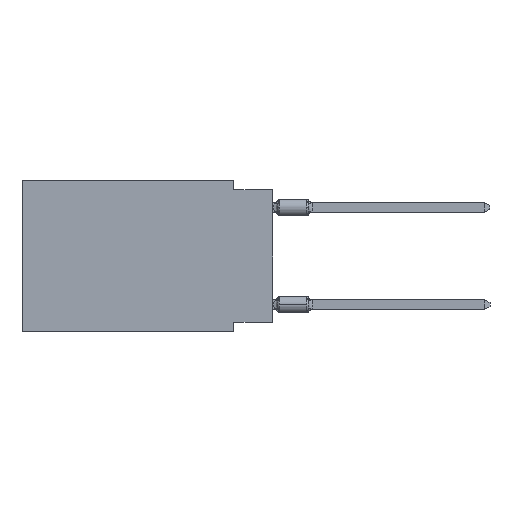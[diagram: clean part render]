
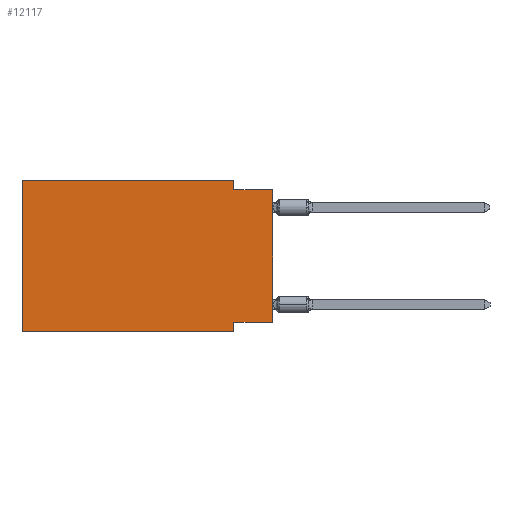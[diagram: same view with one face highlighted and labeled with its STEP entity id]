
A CAD part, left-side view. The second image highlights one B-rep face of the part: STEP entity #12117.
In plain terms, the highlighted planar face has unit normal (-1, 0, 0).
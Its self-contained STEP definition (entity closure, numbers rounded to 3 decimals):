
#54 = VERTEX_POINT ( 'NONE', #26732 ) ;
#307 = VECTOR ( 'NONE', #13949, 1000. ) ;
#312 = CARTESIAN_POINT ( 'NONE',  ( 0., 0., -0.635 ) ) ;
#719 = VERTEX_POINT ( 'NONE', #14793 ) ;
#890 = LINE ( 'NONE', #18001, #26978 ) ;
#1674 = ORIENTED_EDGE ( 'NONE', *, *, #17849, .F. ) ;
#1711 = CARTESIAN_POINT ( 'NONE',  ( 0., 16.383, 0. ) ) ;
#2446 = LINE ( 'NONE', #312, #4805 ) ;
#3516 = DIRECTION ( 'NONE',  ( 0., -1., 0. ) ) ;
#4029 = DIRECTION ( 'NONE',  ( 0., 0., -1. ) ) ;
#4164 = EDGE_CURVE ( 'NONE', #10334, #15615, #7553, .T. ) ;
#4517 = LINE ( 'NONE', #13297, #17828 ) ;
#4805 = VECTOR ( 'NONE', #6915, 1000. ) ;
#5152 = CARTESIAN_POINT ( 'NONE',  ( 0., 0., -9.271 ) ) ;
#6204 = EDGE_CURVE ( 'NONE', #11853, #719, #19268, .T. ) ;
#6274 = VECTOR ( 'NONE', #3516, 1000. ) ;
#6915 = DIRECTION ( 'NONE',  ( 0., -1., 0. ) ) ;
#6929 = EDGE_CURVE ( 'NONE', #15615, #13027, #2446, .T. ) ;
#7408 = CARTESIAN_POINT ( 'NONE',  ( 0., 2.54, 0. ) ) ;
#7469 = ORIENTED_EDGE ( 'NONE', *, *, #23683, .F. ) ;
#7553 = LINE ( 'NONE', #7408, #8108 ) ;
#7963 = VECTOR ( 'NONE', #11773, 1000. ) ;
#8108 = VECTOR ( 'NONE', #25075, 1000. ) ;
#8373 = ORIENTED_EDGE ( 'NONE', *, *, #25994, .F. ) ;
#9087 = CARTESIAN_POINT ( 'NONE',  ( 0., 2.54, -0.635 ) ) ;
#9780 = ORIENTED_EDGE ( 'NONE', *, *, #23783, .T. ) ;
#9837 = VERTEX_POINT ( 'NONE', #20616 ) ;
#10334 = VERTEX_POINT ( 'NONE', #22895 ) ;
#10421 = LINE ( 'NONE', #12288, #6274 ) ;
#10501 = DIRECTION ( 'NONE',  ( 1., 0., 0. ) ) ;
#11773 = DIRECTION ( 'NONE',  ( 0., 1., 0. ) ) ;
#11853 = VERTEX_POINT ( 'NONE', #26566 ) ;
#12117 = ADVANCED_FACE ( 'NONE', ( #21418 ), #12659, .F. ) ;
#12288 = CARTESIAN_POINT ( 'NONE',  ( 0., 16.383, 0. ) ) ;
#12659 = PLANE ( 'NONE',  #20421 ) ;
#13027 = VERTEX_POINT ( 'NONE', #13121 ) ;
#13121 = CARTESIAN_POINT ( 'NONE',  ( 0., 0., -0.635 ) ) ;
#13297 = CARTESIAN_POINT ( 'NONE',  ( 0., 16.383, 0. ) ) ;
#13458 = VECTOR ( 'NONE', #25838, 1000. ) ;
#13949 = DIRECTION ( 'NONE',  ( 0., 0., -1. ) ) ;
#14280 = EDGE_CURVE ( 'NONE', #9837, #719, #15811, .T. ) ;
#14793 = CARTESIAN_POINT ( 'NONE',  ( 0., 2.54, -9.906 ) ) ;
#15026 = CARTESIAN_POINT ( 'NONE',  ( 0., 0., -9.271 ) ) ;
#15615 = VERTEX_POINT ( 'NONE', #9087 ) ;
#15811 = LINE ( 'NONE', #20252, #307 ) ;
#17111 = CARTESIAN_POINT ( 'NONE',  ( 0., 16.383, -9.906 ) ) ;
#17828 = VECTOR ( 'NONE', #22043, 1000. ) ;
#17849 = EDGE_CURVE ( 'NONE', #20034, #9837, #18252, .T. ) ;
#18001 = CARTESIAN_POINT ( 'NONE',  ( 0., 0., 0. ) ) ;
#18252 = LINE ( 'NONE', #5152, #7963 ) ;
#19268 = LINE ( 'NONE', #17111, #13458 ) ;
#20034 = VERTEX_POINT ( 'NONE', #15026 ) ;
#20252 = CARTESIAN_POINT ( 'NONE',  ( 0., 2.54, -9.906 ) ) ;
#20421 = AXIS2_PLACEMENT_3D ( 'NONE', #1711, #10501, #4029 ) ;
#20616 = CARTESIAN_POINT ( 'NONE',  ( 0., 2.54, -9.271 ) ) ;
#20811 = EDGE_LOOP ( 'NONE', ( #9780, #25500, #24382, #8373, #7469, #23634, #21409, #1674 ) ) ;
#21409 = ORIENTED_EDGE ( 'NONE', *, *, #14280, .F. ) ;
#21418 = FACE_OUTER_BOUND ( 'NONE', #20811, .T. ) ;
#22043 = DIRECTION ( 'NONE',  ( 0., 0., 1. ) ) ;
#22895 = CARTESIAN_POINT ( 'NONE',  ( 0., 2.54, 0. ) ) ;
#23634 = ORIENTED_EDGE ( 'NONE', *, *, #6204, .T. ) ;
#23683 = EDGE_CURVE ( 'NONE', #11853, #54, #4517, .T. ) ;
#23783 = EDGE_CURVE ( 'NONE', #20034, #13027, #890, .T. ) ;
#24382 = ORIENTED_EDGE ( 'NONE', *, *, #4164, .F. ) ;
#25075 = DIRECTION ( 'NONE',  ( 0., 0., -1. ) ) ;
#25500 = ORIENTED_EDGE ( 'NONE', *, *, #6929, .F. ) ;
#25838 = DIRECTION ( 'NONE',  ( 0., -1., 0. ) ) ;
#25994 = EDGE_CURVE ( 'NONE', #54, #10334, #10421, .T. ) ;
#26566 = CARTESIAN_POINT ( 'NONE',  ( 0., 16.383, -9.906 ) ) ;
#26725 = DIRECTION ( 'NONE',  ( 0., 0., 1. ) ) ;
#26732 = CARTESIAN_POINT ( 'NONE',  ( 0., 16.383, 0. ) ) ;
#26978 = VECTOR ( 'NONE', #26725, 1000. ) ;
